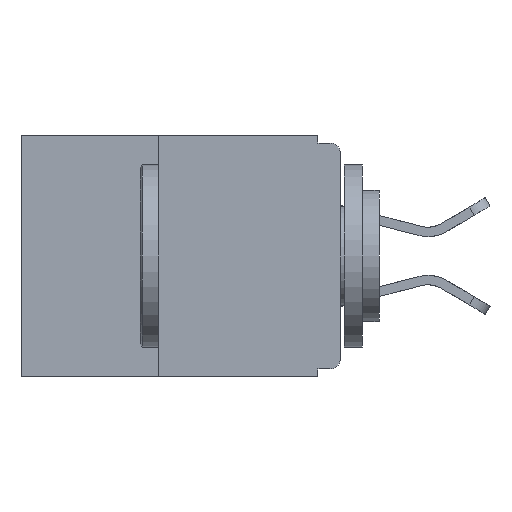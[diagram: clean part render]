
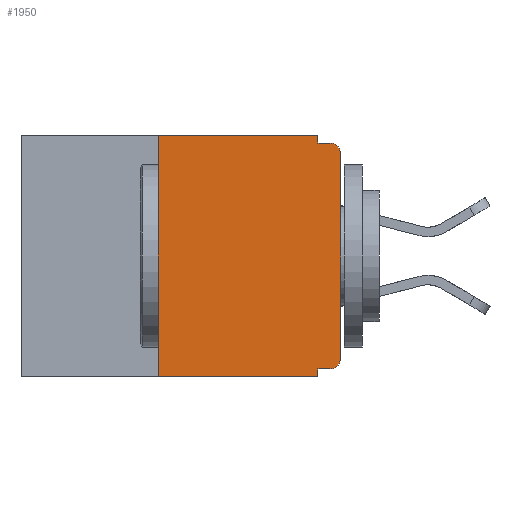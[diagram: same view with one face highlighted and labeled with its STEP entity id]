
A CAD part, left-side view. The second image highlights one B-rep face of the part: STEP entity #1950.
In plain terms, the highlighted planar face has unit normal (-1, 0, 0).
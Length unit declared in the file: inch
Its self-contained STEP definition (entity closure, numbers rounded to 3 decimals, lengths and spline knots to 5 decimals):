
#123 = CARTESIAN_POINT ( 'NONE',  ( 0., 0.015, -0.32 ) ) ;
#208 = LINE ( 'NONE', #903, #10856 ) ;
#275 = CARTESIAN_POINT ( 'NONE',  ( 0., 0.015, -0.01 ) ) ;
#358 = DIRECTION ( 'NONE',  ( 0., -1., 0. ) ) ;
#871 = ORIENTED_EDGE ( 'NONE', *, *, #10385, .F. ) ;
#903 = CARTESIAN_POINT ( 'NONE',  ( 0., 0.437, 0. ) ) ;
#915 = DIRECTION ( 'NONE',  ( 0., -1., 0. ) ) ;
#1152 = VERTEX_POINT ( 'NONE', #16382 ) ;
#1680 = CARTESIAN_POINT ( 'NONE',  ( 0., 0.031, 0. ) ) ;
#1795 = CARTESIAN_POINT ( 'NONE',  ( 0., 0.031, 0. ) ) ;
#1950 = ADVANCED_FACE ( 'NONE', ( #2056 ), #14462, .F. ) ;
#2056 = FACE_OUTER_BOUND ( 'NONE', #4336, .T. ) ;
#2194 = VERTEX_POINT ( 'NONE', #12619 ) ;
#2227 = DIRECTION ( 'NONE',  ( 0., 0., -1. ) ) ;
#2388 = CARTESIAN_POINT ( 'NONE',  ( 0., 0., 0. ) ) ;
#2449 = CARTESIAN_POINT ( 'NONE',  ( 0., 0.031, -0.01 ) ) ;
#2459 = LINE ( 'NONE', #11034, #6085 ) ;
#2553 = VERTEX_POINT ( 'NONE', #15279 ) ;
#3751 = CARTESIAN_POINT ( 'NONE',  ( 0., 0., -0.01 ) ) ;
#4336 = EDGE_LOOP ( 'NONE', ( #7499, #7053, #6741, #6443, #6223, #5430, #4748, #5003, #871, #12522 ) ) ;
#4387 = DIRECTION ( 'NONE',  ( 0., 0., 1. ) ) ;
#4448 = CARTESIAN_POINT ( 'NONE',  ( 0., 0.25, -0.33 ) ) ;
#4556 = DIRECTION ( 'NONE',  ( -1., 0., 0. ) ) ;
#4670 = VERTEX_POINT ( 'NONE', #123 ) ;
#4748 = ORIENTED_EDGE ( 'NONE', *, *, #13695, .T. ) ;
#5003 = ORIENTED_EDGE ( 'NONE', *, *, #11551, .F. ) ;
#5079 = VERTEX_POINT ( 'NONE', #14422 ) ;
#5144 = LINE ( 'NONE', #3751, #11742 ) ;
#5430 = ORIENTED_EDGE ( 'NONE', *, *, #6289, .F. ) ;
#5488 = LINE ( 'NONE', #10221, #12457 ) ;
#5707 = EDGE_CURVE ( 'NONE', #4670, #6711, #8478, .T. ) ;
#5750 = AXIS2_PLACEMENT_3D ( 'NONE', #12444, #4556, #13730 ) ;
#5812 = CIRCLE ( 'NONE', #5750, 0.015 ) ;
#6085 = VECTOR ( 'NONE', #358, 39.37008 ) ;
#6223 = ORIENTED_EDGE ( 'NONE', *, *, #6600, .F. ) ;
#6289 = EDGE_CURVE ( 'NONE', #2194, #6846, #14827, .T. ) ;
#6439 = VERTEX_POINT ( 'NONE', #2449 ) ;
#6443 = ORIENTED_EDGE ( 'NONE', *, *, #11956, .F. ) ;
#6449 = DIRECTION ( 'NONE',  ( 0., 0., 1. ) ) ;
#6600 = EDGE_CURVE ( 'NONE', #6846, #7261, #208, .T. ) ;
#6711 = VERTEX_POINT ( 'NONE', #14447 ) ;
#6741 = ORIENTED_EDGE ( 'NONE', *, *, #10996, .F. ) ;
#6846 = VERTEX_POINT ( 'NONE', #13375 ) ;
#7053 = ORIENTED_EDGE ( 'NONE', *, *, #10726, .T. ) ;
#7261 = VERTEX_POINT ( 'NONE', #1795 ) ;
#7499 = ORIENTED_EDGE ( 'NONE', *, *, #12893, .T. ) ;
#7717 = VECTOR ( 'NONE', #10427, 39.37008 ) ;
#8417 = VECTOR ( 'NONE', #6449, 39.37008 ) ;
#8478 = CIRCLE ( 'NONE', #10548, 0.015 ) ;
#8721 = DIRECTION ( 'NONE',  ( 0., 0., -1. ) ) ;
#8724 = DIRECTION ( 'NONE',  ( -1., 0., 0. ) ) ;
#8742 = CARTESIAN_POINT ( 'NONE',  ( 0., 0.015, -0.305 ) ) ;
#9022 = VECTOR ( 'NONE', #12301, 39.37008 ) ;
#9225 = AXIS2_PLACEMENT_3D ( 'NONE', #12839, #10795, #15416 ) ;
#10221 = CARTESIAN_POINT ( 'NONE',  ( 0., 0.031, -0.33 ) ) ;
#10385 = EDGE_CURVE ( 'NONE', #4670, #2553, #14513, .T. ) ;
#10427 = DIRECTION ( 'NONE',  ( 0., 1., 0. ) ) ;
#10548 = AXIS2_PLACEMENT_3D ( 'NONE', #8742, #8724, #8721 ) ;
#10726 = EDGE_CURVE ( 'NONE', #5079, #11931, #5812, .T. ) ;
#10795 = DIRECTION ( 'NONE',  ( 1., 0., 0. ) ) ;
#10856 = VECTOR ( 'NONE', #915, 39.37008 ) ;
#10996 = EDGE_CURVE ( 'NONE', #6439, #11931, #5144, .T. ) ;
#11034 = CARTESIAN_POINT ( 'NONE',  ( 0., 0.437, -0.33 ) ) ;
#11477 = VECTOR ( 'NONE', #4387, 39.37008 ) ;
#11551 = EDGE_CURVE ( 'NONE', #2553, #1152, #5488, .T. ) ;
#11715 = DIRECTION ( 'NONE',  ( 0., -1., 0. ) ) ;
#11742 = VECTOR ( 'NONE', #11715, 39.37008 ) ;
#11931 = VERTEX_POINT ( 'NONE', #275 ) ;
#11956 = EDGE_CURVE ( 'NONE', #7261, #6439, #15723, .T. ) ;
#12301 = DIRECTION ( 'NONE',  ( 0., 0., -1. ) ) ;
#12444 = CARTESIAN_POINT ( 'NONE',  ( 0., 0.015, -0.025 ) ) ;
#12457 = VECTOR ( 'NONE', #2227, 39.37008 ) ;
#12522 = ORIENTED_EDGE ( 'NONE', *, *, #5707, .T. ) ;
#12619 = CARTESIAN_POINT ( 'NONE',  ( 0., 0.25, -0.33 ) ) ;
#12839 = CARTESIAN_POINT ( 'NONE',  ( 0., 0.437, 0. ) ) ;
#12893 = EDGE_CURVE ( 'NONE', #6711, #5079, #15531, .T. ) ;
#13375 = CARTESIAN_POINT ( 'NONE',  ( 0., 0.25, 0. ) ) ;
#13695 = EDGE_CURVE ( 'NONE', #2194, #1152, #2459, .T. ) ;
#13730 = DIRECTION ( 'NONE',  ( 0., 0., -1. ) ) ;
#14422 = CARTESIAN_POINT ( 'NONE',  ( 0., 0., -0.025 ) ) ;
#14447 = CARTESIAN_POINT ( 'NONE',  ( 0., 0., -0.305 ) ) ;
#14462 = PLANE ( 'NONE',  #9225 ) ;
#14513 = LINE ( 'NONE', #15431, #7717 ) ;
#14827 = LINE ( 'NONE', #4448, #11477 ) ;
#15279 = CARTESIAN_POINT ( 'NONE',  ( 0., 0.031, -0.32 ) ) ;
#15416 = DIRECTION ( 'NONE',  ( 0., 0., -1. ) ) ;
#15431 = CARTESIAN_POINT ( 'NONE',  ( 0., 0., -0.32 ) ) ;
#15531 = LINE ( 'NONE', #2388, #8417 ) ;
#15723 = LINE ( 'NONE', #1680, #9022 ) ;
#16382 = CARTESIAN_POINT ( 'NONE',  ( 0., 0.031, -0.33 ) ) ;
